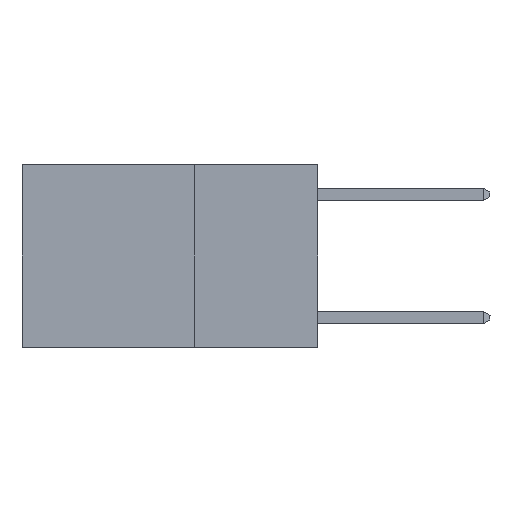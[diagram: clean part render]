
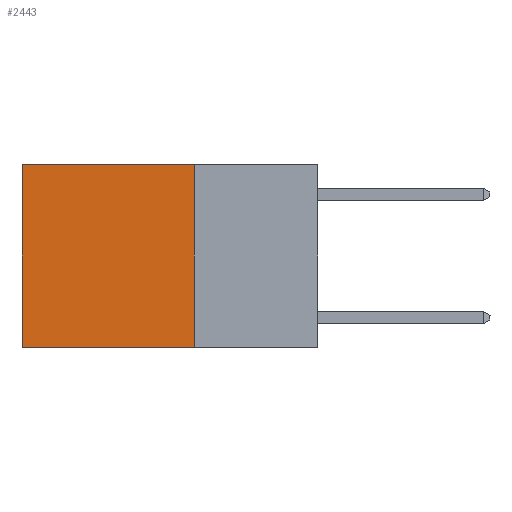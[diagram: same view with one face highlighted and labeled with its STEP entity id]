
A CAD part, left-side view. The second image highlights one B-rep face of the part: STEP entity #2443.
In plain terms, the highlighted planar face has unit normal (-1, 0, 0).
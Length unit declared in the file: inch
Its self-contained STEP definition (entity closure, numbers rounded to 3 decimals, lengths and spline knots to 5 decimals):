
#275 = VERTEX_POINT ( 'NONE', #5135 ) ;
#354 = VECTOR ( 'NONE', #9537, 39.37008 ) ;
#416 = EDGE_CURVE ( 'NONE', #8969, #275, #11899, .T. ) ;
#1355 = DIRECTION ( 'NONE',  ( 0., 0., -1. ) ) ;
#1463 = PLANE ( 'NONE',  #7921 ) ;
#1538 = VERTEX_POINT ( 'NONE', #7089 ) ;
#1678 = DIRECTION ( 'NONE',  ( 0., 0., -1. ) ) ;
#1694 = CARTESIAN_POINT ( 'NONE',  ( 0.2625, 0.25, 0. ) ) ;
#1756 = LINE ( 'NONE', #1694, #5117 ) ;
#2443 = ADVANCED_FACE ( 'NONE', ( #6692 ), #1463, .F. ) ;
#2824 = LINE ( 'NONE', #13526, #9023 ) ;
#3553 = CARTESIAN_POINT ( 'NONE',  ( 0.2625, 0.25, -0.37 ) ) ;
#4130 = LINE ( 'NONE', #4734, #354 ) ;
#4734 = CARTESIAN_POINT ( 'NONE',  ( 0.2625, 0.6, 0. ) ) ;
#5107 = DIRECTION ( 'NONE',  ( 1., 0., 0. ) ) ;
#5117 = VECTOR ( 'NONE', #13805, 39.37008 ) ;
#5135 = CARTESIAN_POINT ( 'NONE',  ( 0.2625, 0.6, -0.37 ) ) ;
#5212 = CARTESIAN_POINT ( 'NONE',  ( 0.2625, 0.25, 0. ) ) ;
#6388 = ORIENTED_EDGE ( 'NONE', *, *, #15331, .T. ) ;
#6692 = FACE_OUTER_BOUND ( 'NONE', #15196, .T. ) ;
#6760 = ORIENTED_EDGE ( 'NONE', *, *, #11159, .F. ) ;
#7089 = CARTESIAN_POINT ( 'NONE',  ( 0.2625, 0.6, 0. ) ) ;
#7233 = VERTEX_POINT ( 'NONE', #14862 ) ;
#7921 = AXIS2_PLACEMENT_3D ( 'NONE', #5212, #5107, #1678 ) ;
#8582 = ORIENTED_EDGE ( 'NONE', *, *, #11607, .T. ) ;
#8653 = ORIENTED_EDGE ( 'NONE', *, *, #416, .F. ) ;
#8969 = VERTEX_POINT ( 'NONE', #3553 ) ;
#9023 = VECTOR ( 'NONE', #1355, 39.37008 ) ;
#9537 = DIRECTION ( 'NONE',  ( 0., 0., -1. ) ) ;
#10337 = VECTOR ( 'NONE', #12718, 39.37008 ) ;
#11159 = EDGE_CURVE ( 'NONE', #7233, #8969, #2824, .T. ) ;
#11607 = EDGE_CURVE ( 'NONE', #1538, #275, #4130, .T. ) ;
#11899 = LINE ( 'NONE', #15240, #10337 ) ;
#12718 = DIRECTION ( 'NONE',  ( 0., 1., 0. ) ) ;
#13526 = CARTESIAN_POINT ( 'NONE',  ( 0.2625, 0.25, 0. ) ) ;
#13805 = DIRECTION ( 'NONE',  ( 0., 1., 0. ) ) ;
#14862 = CARTESIAN_POINT ( 'NONE',  ( 0.2625, 0.25, 0. ) ) ;
#15196 = EDGE_LOOP ( 'NONE', ( #8582, #8653, #6760, #6388 ) ) ;
#15240 = CARTESIAN_POINT ( 'NONE',  ( 0.2625, 0.25, -0.37 ) ) ;
#15331 = EDGE_CURVE ( 'NONE', #7233, #1538, #1756, .T. ) ;
